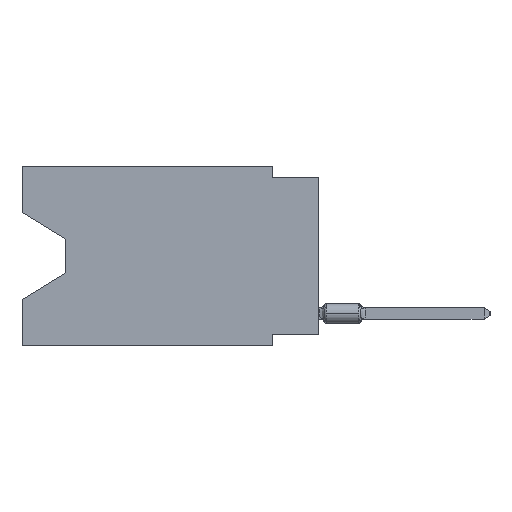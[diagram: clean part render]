
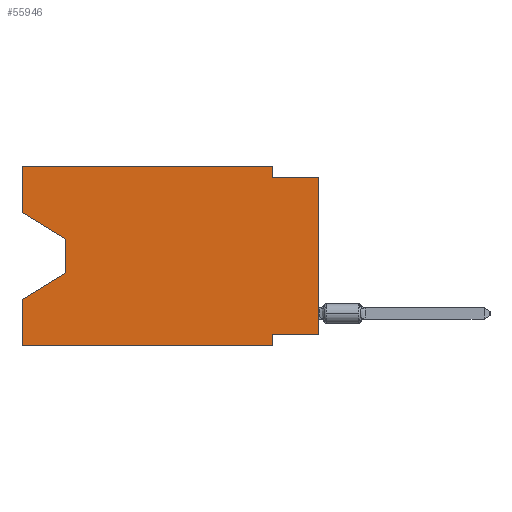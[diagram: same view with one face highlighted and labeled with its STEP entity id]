
A CAD part, left-side view. The second image highlights one B-rep face of the part: STEP entity #55946.
In plain terms, the highlighted planar face has unit normal (-1, 0, 0).
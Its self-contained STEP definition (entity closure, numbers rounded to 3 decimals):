
#335 = EDGE_LOOP ( 'NONE', ( #9116, #24968, #61621, #63519, #41056, #2791, #54788, #65540, #59541, #50156, #63627, #19555 ) ) ;
#807 = VERTEX_POINT ( 'NONE', #16256 ) ;
#2287 = AXIS2_PLACEMENT_3D ( 'NONE', #31281, #11455, #31950 ) ;
#2791 = ORIENTED_EDGE ( 'NONE', *, *, #64298, .F. ) ;
#4795 = VECTOR ( 'NONE', #34078, 1000. ) ;
#4976 = FACE_OUTER_BOUND ( 'NONE', #335, .T. ) ;
#6367 = LINE ( 'NONE', #21755, #19774 ) ;
#6731 = VERTEX_POINT ( 'NONE', #56639 ) ;
#7177 = LINE ( 'NONE', #43402, #14229 ) ;
#7967 = CARTESIAN_POINT ( 'NONE',  ( 0., 13.97, -5.893 ) ) ;
#8055 = DIRECTION ( 'NONE',  ( 0., 0., -1. ) ) ;
#9003 = VECTOR ( 'NONE', #8055, 1000. ) ;
#9116 = ORIENTED_EDGE ( 'NONE', *, *, #64528, .T. ) ;
#10011 = DIRECTION ( 'NONE',  ( 0., -1., 0. ) ) ;
#10337 = EDGE_CURVE ( 'NONE', #45023, #32036, #6367, .T. ) ;
#10375 = CARTESIAN_POINT ( 'NONE',  ( 0., 16.383, 0. ) ) ;
#10403 = DIRECTION ( 'NONE',  ( 0., 0., 1. ) ) ;
#10541 = CARTESIAN_POINT ( 'NONE',  ( 0., 13.97, -5.893 ) ) ;
#11455 = DIRECTION ( 'NONE',  ( 1., 0., 0. ) ) ;
#12173 = LINE ( 'NONE', #65467, #9003 ) ;
#13270 = VERTEX_POINT ( 'NONE', #20888 ) ;
#13284 = VERTEX_POINT ( 'NONE', #20215 ) ;
#13436 = LINE ( 'NONE', #7967, #29711 ) ;
#14229 = VECTOR ( 'NONE', #48870, 1000. ) ;
#14610 = VECTOR ( 'NONE', #10403, 1000. ) ;
#15348 = EDGE_CURVE ( 'NONE', #13270, #13284, #31243, .T. ) ;
#16000 = CARTESIAN_POINT ( 'NONE',  ( 0., 16.383, -7.36 ) ) ;
#16213 = VERTEX_POINT ( 'NONE', #45194 ) ;
#16247 = CARTESIAN_POINT ( 'NONE',  ( 0., 16.383, 0. ) ) ;
#16256 = CARTESIAN_POINT ( 'NONE',  ( 0., 16.383, 0. ) ) ;
#16756 = CARTESIAN_POINT ( 'NONE',  ( 0., 2.54, -9.906 ) ) ;
#18215 = CARTESIAN_POINT ( 'NONE',  ( 0., 2.54, 0. ) ) ;
#19036 = VECTOR ( 'NONE', #57537, 1000. ) ;
#19555 = ORIENTED_EDGE ( 'NONE', *, *, #57660, .F. ) ;
#19774 = VECTOR ( 'NONE', #57658, 1000. ) ;
#20126 = EDGE_CURVE ( 'NONE', #13270, #6731, #30120, .T. ) ;
#20215 = CARTESIAN_POINT ( 'NONE',  ( 0., 0., -0.635 ) ) ;
#20888 = CARTESIAN_POINT ( 'NONE',  ( 0., 0., -9.271 ) ) ;
#21224 = DIRECTION ( 'NONE',  ( 0., 0., -1. ) ) ;
#21607 = CARTESIAN_POINT ( 'NONE',  ( 0., 0., -0.635 ) ) ;
#21713 = VECTOR ( 'NONE', #55103, 1000. ) ;
#21755 = CARTESIAN_POINT ( 'NONE',  ( 0., 16.383, 0. ) ) ;
#22861 = VERTEX_POINT ( 'NONE', #18215 ) ;
#24156 = LINE ( 'NONE', #39214, #4795 ) ;
#24952 = VERTEX_POINT ( 'NONE', #55111 ) ;
#24968 = ORIENTED_EDGE ( 'NONE', *, *, #46775, .T. ) ;
#26340 = VERTEX_POINT ( 'NONE', #65517 ) ;
#29148 = DIRECTION ( 'NONE',  ( 0., 0.855, -0.519 ) ) ;
#29480 = CARTESIAN_POINT ( 'NONE',  ( 0., 16.383, -9.906 ) ) ;
#29711 = VECTOR ( 'NONE', #29148, 1000. ) ;
#30120 = LINE ( 'NONE', #60210, #21713 ) ;
#31243 = LINE ( 'NONE', #47298, #14610 ) ;
#31281 = CARTESIAN_POINT ( 'NONE',  ( 0., 16.383, 0. ) ) ;
#31950 = DIRECTION ( 'NONE',  ( 0., 0., -1. ) ) ;
#32036 = VERTEX_POINT ( 'NONE', #16000 ) ;
#32206 = LINE ( 'NONE', #21607, #38145 ) ;
#33217 = EDGE_CURVE ( 'NONE', #16213, #13284, #32206, .T. ) ;
#34078 = DIRECTION ( 'NONE',  ( 0., 0., -1. ) ) ;
#34391 = LINE ( 'NONE', #45989, #46927 ) ;
#34907 = VECTOR ( 'NONE', #21224, 1000. ) ;
#36331 = LINE ( 'NONE', #10375, #19036 ) ;
#38145 = VECTOR ( 'NONE', #10011, 1000. ) ;
#39087 = EDGE_CURVE ( 'NONE', #22861, #16213, #12173, .T. ) ;
#39214 = CARTESIAN_POINT ( 'NONE',  ( 0., 13.97, -4.013 ) ) ;
#41056 = ORIENTED_EDGE ( 'NONE', *, *, #63854, .T. ) ;
#43402 = CARTESIAN_POINT ( 'NONE',  ( 0., 16.383, -2.546 ) ) ;
#44856 = EDGE_CURVE ( 'NONE', #64703, #32036, #13436, .T. ) ;
#45023 = VERTEX_POINT ( 'NONE', #29480 ) ;
#45194 = CARTESIAN_POINT ( 'NONE',  ( 0., 2.54, -0.635 ) ) ;
#45989 = CARTESIAN_POINT ( 'NONE',  ( 0., 16.383, -9.906 ) ) ;
#46775 = EDGE_CURVE ( 'NONE', #24952, #64703, #24156, .T. ) ;
#46927 = VECTOR ( 'NONE', #60687, 1000. ) ;
#47298 = CARTESIAN_POINT ( 'NONE',  ( 0., 0., 0. ) ) ;
#48870 = DIRECTION ( 'NONE',  ( 0., -0.855, -0.519 ) ) ;
#50156 = ORIENTED_EDGE ( 'NONE', *, *, #39087, .F. ) ;
#52651 = LINE ( 'NONE', #16756, #34907 ) ;
#52817 = DIRECTION ( 'NONE',  ( 0., -1., 0. ) ) ;
#54518 = VERTEX_POINT ( 'NONE', #60336 ) ;
#54788 = ORIENTED_EDGE ( 'NONE', *, *, #20126, .F. ) ;
#55103 = DIRECTION ( 'NONE',  ( 0., 1., 0. ) ) ;
#55111 = CARTESIAN_POINT ( 'NONE',  ( 0., 13.97, -4.013 ) ) ;
#55946 = ADVANCED_FACE ( 'NONE', ( #4976 ), #62370, .F. ) ;
#56639 = CARTESIAN_POINT ( 'NONE',  ( 0., 2.54, -9.271 ) ) ;
#57437 = VECTOR ( 'NONE', #52817, 1000. ) ;
#57537 = DIRECTION ( 'NONE',  ( 0., 0., 1. ) ) ;
#57658 = DIRECTION ( 'NONE',  ( 0., 0., 1. ) ) ;
#57660 = EDGE_CURVE ( 'NONE', #54518, #807, #36331, .T. ) ;
#59158 = EDGE_CURVE ( 'NONE', #807, #22861, #63045, .T. ) ;
#59541 = ORIENTED_EDGE ( 'NONE', *, *, #33217, .F. ) ;
#60210 = CARTESIAN_POINT ( 'NONE',  ( 0., 0., -9.271 ) ) ;
#60336 = CARTESIAN_POINT ( 'NONE',  ( 0., 16.383, -2.546 ) ) ;
#60687 = DIRECTION ( 'NONE',  ( 0., -1., 0. ) ) ;
#61621 = ORIENTED_EDGE ( 'NONE', *, *, #44856, .T. ) ;
#62370 = PLANE ( 'NONE',  #2287 ) ;
#63045 = LINE ( 'NONE', #16247, #57437 ) ;
#63519 = ORIENTED_EDGE ( 'NONE', *, *, #10337, .F. ) ;
#63627 = ORIENTED_EDGE ( 'NONE', *, *, #59158, .F. ) ;
#63854 = EDGE_CURVE ( 'NONE', #45023, #26340, #34391, .T. ) ;
#64298 = EDGE_CURVE ( 'NONE', #6731, #26340, #52651, .T. ) ;
#64528 = EDGE_CURVE ( 'NONE', #54518, #24952, #7177, .T. ) ;
#64703 = VERTEX_POINT ( 'NONE', #10541 ) ;
#65467 = CARTESIAN_POINT ( 'NONE',  ( 0., 2.54, 0. ) ) ;
#65517 = CARTESIAN_POINT ( 'NONE',  ( 0., 2.54, -9.906 ) ) ;
#65540 = ORIENTED_EDGE ( 'NONE', *, *, #15348, .T. ) ;
